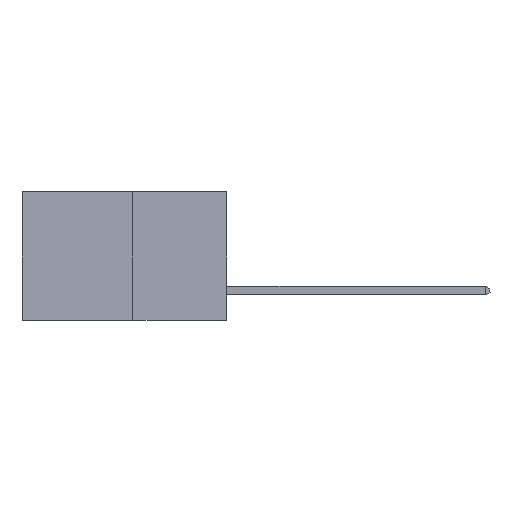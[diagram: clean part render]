
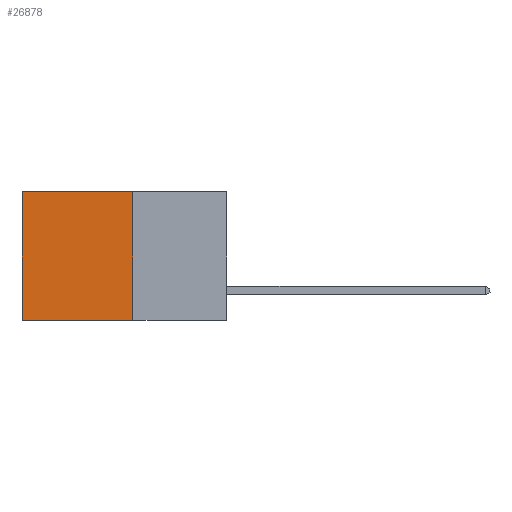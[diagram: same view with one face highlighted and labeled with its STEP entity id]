
A CAD part, left-side view. The second image highlights one B-rep face of the part: STEP entity #26878.
In plain terms, the highlighted planar face has unit normal (-1, 0, 0).
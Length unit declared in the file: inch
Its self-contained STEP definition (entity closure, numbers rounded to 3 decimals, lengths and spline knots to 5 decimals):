
#2107 = ORIENTED_EDGE ( 'NONE', *, *, #5329, .F. ) ;
#3768 = VERTEX_POINT ( 'NONE', #28465 ) ;
#5168 = EDGE_CURVE ( 'NONE', #3768, #25868, #22603, .T. ) ;
#5209 = ORIENTED_EDGE ( 'NONE', *, *, #28464, .T. ) ;
#5329 = EDGE_CURVE ( 'NONE', #23040, #16416, #5444, .T. ) ;
#5444 = LINE ( 'NONE', #19204, #29904 ) ;
#5690 = DIRECTION ( 'NONE',  ( 0., 1., 0. ) ) ;
#9288 = DIRECTION ( 'NONE',  ( 1., 0., 0. ) ) ;
#9724 = VECTOR ( 'NONE', #10953, 39.37008 ) ;
#9959 = VECTOR ( 'NONE', #21222, 39.37008 ) ;
#10953 = DIRECTION ( 'NONE',  ( 0., 1., 0. ) ) ;
#11053 = AXIS2_PLACEMENT_3D ( 'NONE', #11643, #9288, #25921 ) ;
#11643 = CARTESIAN_POINT ( 'NONE',  ( 0.277, 0.27, -0.37 ) ) ;
#13430 = CARTESIAN_POINT ( 'NONE',  ( 0.277, 0.27, -0.37 ) ) ;
#15198 = CARTESIAN_POINT ( 'NONE',  ( 0.277, 0.27, 0. ) ) ;
#15208 = CARTESIAN_POINT ( 'NONE',  ( 0.277, 0.59, -0.37 ) ) ;
#15332 = LINE ( 'NONE', #15712, #9724 ) ;
#15361 = VECTOR ( 'NONE', #5690, 39.37008 ) ;
#15712 = CARTESIAN_POINT ( 'NONE',  ( 0.277, 0.27, -0.37 ) ) ;
#16416 = VERTEX_POINT ( 'NONE', #13430 ) ;
#18582 = EDGE_CURVE ( 'NONE', #16416, #25868, #15332, .T. ) ;
#19106 = DIRECTION ( 'NONE',  ( 0., 0., -1. ) ) ;
#19204 = CARTESIAN_POINT ( 'NONE',  ( 0.277, 0.27, -0.37 ) ) ;
#20129 = ORIENTED_EDGE ( 'NONE', *, *, #5168, .T. ) ;
#20465 = EDGE_LOOP ( 'NONE', ( #20129, #21620, #2107, #5209 ) ) ;
#21222 = DIRECTION ( 'NONE',  ( 0., 0., -1. ) ) ;
#21393 = CARTESIAN_POINT ( 'NONE',  ( 0.277, 0.59, -0.37 ) ) ;
#21620 = ORIENTED_EDGE ( 'NONE', *, *, #18582, .F. ) ;
#22603 = LINE ( 'NONE', #21393, #9959 ) ;
#23040 = VERTEX_POINT ( 'NONE', #28669 ) ;
#23548 = PLANE ( 'NONE',  #11053 ) ;
#25868 = VERTEX_POINT ( 'NONE', #15208 ) ;
#25921 = DIRECTION ( 'NONE',  ( 0., 0., -1. ) ) ;
#26878 = ADVANCED_FACE ( 'NONE', ( #26898 ), #23548, .F. ) ;
#26898 = FACE_OUTER_BOUND ( 'NONE', #20465, .T. ) ;
#27915 = LINE ( 'NONE', #15198, #15361 ) ;
#28464 = EDGE_CURVE ( 'NONE', #23040, #3768, #27915, .T. ) ;
#28465 = CARTESIAN_POINT ( 'NONE',  ( 0.277, 0.59, 0. ) ) ;
#28669 = CARTESIAN_POINT ( 'NONE',  ( 0.277, 0.27, 0. ) ) ;
#29904 = VECTOR ( 'NONE', #19106, 39.37008 ) ;
